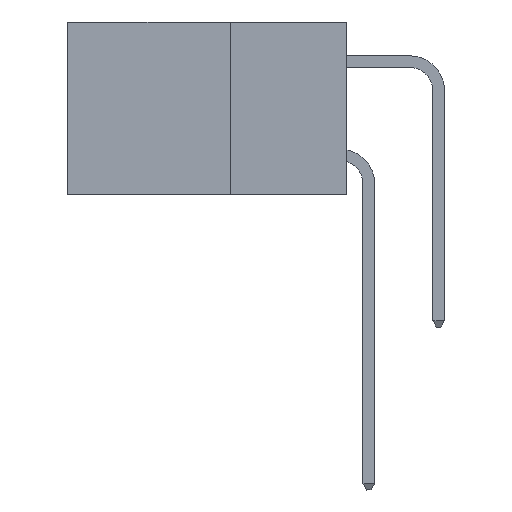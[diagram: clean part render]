
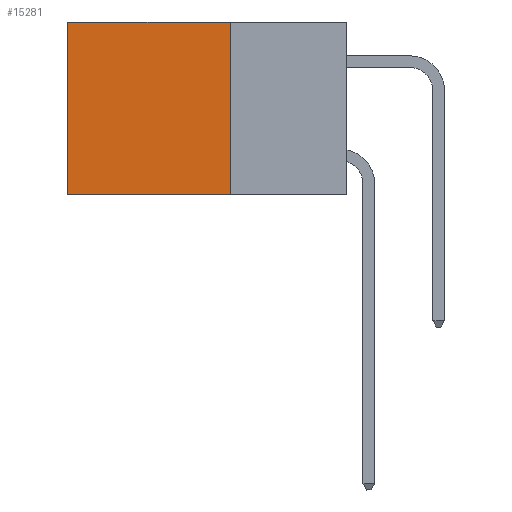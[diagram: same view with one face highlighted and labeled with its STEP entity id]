
A CAD part, left-side view. The second image highlights one B-rep face of the part: STEP entity #15281.
In plain terms, the highlighted planar face has unit normal (-1, 0, 0).
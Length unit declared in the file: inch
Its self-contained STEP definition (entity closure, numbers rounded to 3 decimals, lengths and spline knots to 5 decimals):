
#253 = PLANE ( 'NONE',  #6169 ) ;
#1775 = DIRECTION ( 'NONE',  ( 0., 0., -1. ) ) ;
#2367 = VERTEX_POINT ( 'NONE', #4131 ) ;
#4131 = CARTESIAN_POINT ( 'NONE',  ( 0.2875, 0.6, -0.37 ) ) ;
#4501 = CARTESIAN_POINT ( 'NONE',  ( 0.2875, 0.25, 0. ) ) ;
#4762 = EDGE_CURVE ( 'NONE', #16151, #2367, #20610, .T. ) ;
#6169 = AXIS2_PLACEMENT_3D ( 'NONE', #12875, #16657, #25697 ) ;
#7221 = DIRECTION ( 'NONE',  ( 0., 1., 0. ) ) ;
#8790 = EDGE_CURVE ( 'NONE', #15714, #16151, #36041, .T. ) ;
#11165 = VERTEX_POINT ( 'NONE', #16423 ) ;
#12690 = ORIENTED_EDGE ( 'NONE', *, *, #41502, .F. ) ;
#12875 = CARTESIAN_POINT ( 'NONE',  ( 0.2875, 0.25, 0. ) ) ;
#13653 = ORIENTED_EDGE ( 'NONE', *, *, #14995, .F. ) ;
#14097 = CARTESIAN_POINT ( 'NONE',  ( 0.2875, 0.6, 0. ) ) ;
#14995 = EDGE_CURVE ( 'NONE', #15714, #11165, #20261, .T. ) ;
#15281 = ADVANCED_FACE ( 'NONE', ( #38315 ), #253, .F. ) ;
#15714 = VERTEX_POINT ( 'NONE', #39273 ) ;
#16151 = VERTEX_POINT ( 'NONE', #29517 ) ;
#16423 = CARTESIAN_POINT ( 'NONE',  ( 0.2875, 0.25, -0.37 ) ) ;
#16657 = DIRECTION ( 'NONE',  ( 1., 0., 0. ) ) ;
#18347 = ORIENTED_EDGE ( 'NONE', *, *, #4762, .T. ) ;
#19152 = VECTOR ( 'NONE', #7221, 39.37008 ) ;
#20261 = LINE ( 'NONE', #20695, #25614 ) ;
#20610 = LINE ( 'NONE', #14097, #32918 ) ;
#20695 = CARTESIAN_POINT ( 'NONE',  ( 0.2875, 0.25, 0. ) ) ;
#20934 = VECTOR ( 'NONE', #34535, 39.37008 ) ;
#21690 = CARTESIAN_POINT ( 'NONE',  ( 0.2875, 0.25, -0.37 ) ) ;
#21901 = LINE ( 'NONE', #21690, #20934 ) ;
#22066 = EDGE_LOOP ( 'NONE', ( #18347, #12690, #13653, #30725 ) ) ;
#25614 = VECTOR ( 'NONE', #1775, 39.37008 ) ;
#25697 = DIRECTION ( 'NONE',  ( 0., 0., -1. ) ) ;
#29517 = CARTESIAN_POINT ( 'NONE',  ( 0.2875, 0.6, 0. ) ) ;
#30270 = DIRECTION ( 'NONE',  ( 0., 0., -1. ) ) ;
#30725 = ORIENTED_EDGE ( 'NONE', *, *, #8790, .T. ) ;
#32918 = VECTOR ( 'NONE', #30270, 39.37008 ) ;
#34535 = DIRECTION ( 'NONE',  ( 0., 1., 0. ) ) ;
#36041 = LINE ( 'NONE', #4501, #19152 ) ;
#38315 = FACE_OUTER_BOUND ( 'NONE', #22066, .T. ) ;
#39273 = CARTESIAN_POINT ( 'NONE',  ( 0.2875, 0.25, 0. ) ) ;
#41502 = EDGE_CURVE ( 'NONE', #11165, #2367, #21901, .T. ) ;
